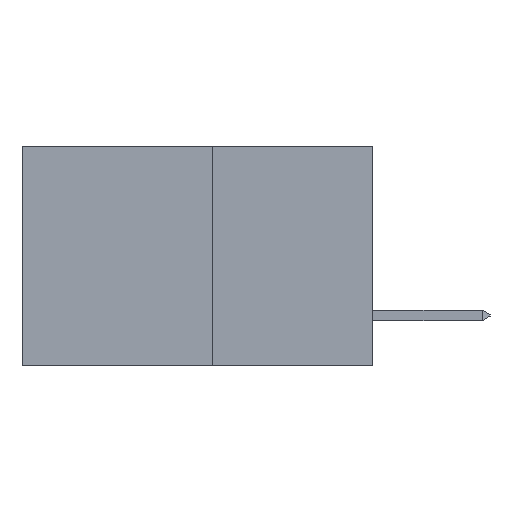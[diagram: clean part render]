
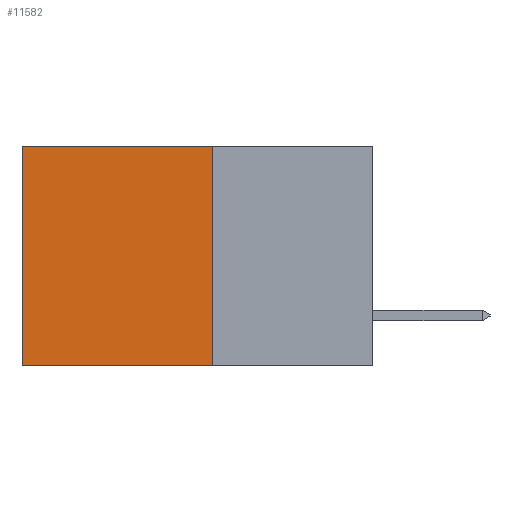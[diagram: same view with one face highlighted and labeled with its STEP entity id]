
A CAD part, left-side view. The second image highlights one B-rep face of the part: STEP entity #11582.
In plain terms, the highlighted planar face has unit normal (-1, 0, 0).
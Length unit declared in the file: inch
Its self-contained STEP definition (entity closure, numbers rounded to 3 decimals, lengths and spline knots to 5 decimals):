
#756 = LINE ( 'NONE', #14622, #6678 ) ;
#1465 = CARTESIAN_POINT ( 'NONE',  ( 0.277, 0.27, -0.37 ) ) ;
#1792 = DIRECTION ( 'NONE',  ( 0., 1., 0. ) ) ;
#2304 = VERTEX_POINT ( 'NONE', #13090 ) ;
#2434 = EDGE_CURVE ( 'NONE', #6235, #2304, #6203, .T. ) ;
#3117 = LINE ( 'NONE', #8479, #8879 ) ;
#3271 = VERTEX_POINT ( 'NONE', #13637 ) ;
#3457 = ORIENTED_EDGE ( 'NONE', *, *, #2434, .F. ) ;
#3772 = VERTEX_POINT ( 'NONE', #4471 ) ;
#3799 = EDGE_CURVE ( 'NONE', #3271, #6235, #3117, .T. ) ;
#4471 = CARTESIAN_POINT ( 'NONE',  ( 0.277, 0.59, 0. ) ) ;
#5091 = ORIENTED_EDGE ( 'NONE', *, *, #6431, .T. ) ;
#5105 = DIRECTION ( 'NONE',  ( 1., 0., 0. ) ) ;
#5497 = AXIS2_PLACEMENT_3D ( 'NONE', #1465, #5105, #13088 ) ;
#5874 = VECTOR ( 'NONE', #10086, 39.37008 ) ;
#6203 = LINE ( 'NONE', #14545, #5874 ) ;
#6235 = VERTEX_POINT ( 'NONE', #12828 ) ;
#6431 = EDGE_CURVE ( 'NONE', #3772, #2304, #11720, .T. ) ;
#6678 = VECTOR ( 'NONE', #1792, 39.37008 ) ;
#6728 = EDGE_CURVE ( 'NONE', #3271, #3772, #756, .T. ) ;
#8296 = VECTOR ( 'NONE', #12546, 39.37008 ) ;
#8479 = CARTESIAN_POINT ( 'NONE',  ( 0.277, 0.27, -0.37 ) ) ;
#8619 = FACE_OUTER_BOUND ( 'NONE', #14550, .T. ) ;
#8879 = VECTOR ( 'NONE', #14834, 39.37008 ) ;
#8977 = ORIENTED_EDGE ( 'NONE', *, *, #3799, .F. ) ;
#10086 = DIRECTION ( 'NONE',  ( 0., 1., 0. ) ) ;
#10744 = ORIENTED_EDGE ( 'NONE', *, *, #6728, .T. ) ;
#11582 = ADVANCED_FACE ( 'NONE', ( #8619 ), #11961, .F. ) ;
#11720 = LINE ( 'NONE', #14706, #8296 ) ;
#11961 = PLANE ( 'NONE',  #5497 ) ;
#12546 = DIRECTION ( 'NONE',  ( 0., 0., -1. ) ) ;
#12828 = CARTESIAN_POINT ( 'NONE',  ( 0.277, 0.27, -0.37 ) ) ;
#13088 = DIRECTION ( 'NONE',  ( 0., 0., -1. ) ) ;
#13090 = CARTESIAN_POINT ( 'NONE',  ( 0.277, 0.59, -0.37 ) ) ;
#13637 = CARTESIAN_POINT ( 'NONE',  ( 0.277, 0.27, 0. ) ) ;
#14545 = CARTESIAN_POINT ( 'NONE',  ( 0.277, 0.27, -0.37 ) ) ;
#14550 = EDGE_LOOP ( 'NONE', ( #5091, #3457, #8977, #10744 ) ) ;
#14622 = CARTESIAN_POINT ( 'NONE',  ( 0.277, 0.27, 0. ) ) ;
#14706 = CARTESIAN_POINT ( 'NONE',  ( 0.277, 0.59, -0.37 ) ) ;
#14834 = DIRECTION ( 'NONE',  ( 0., 0., -1. ) ) ;
